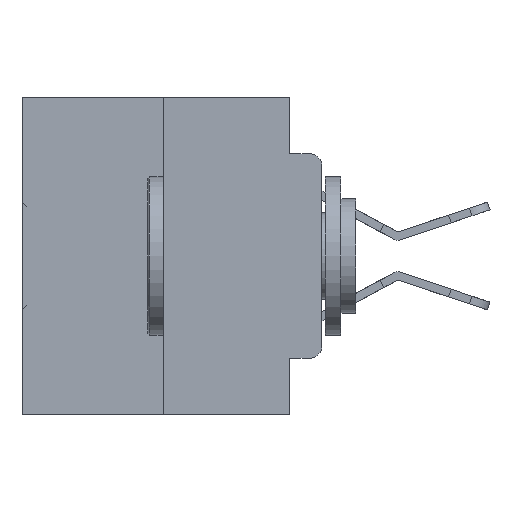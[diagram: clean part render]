
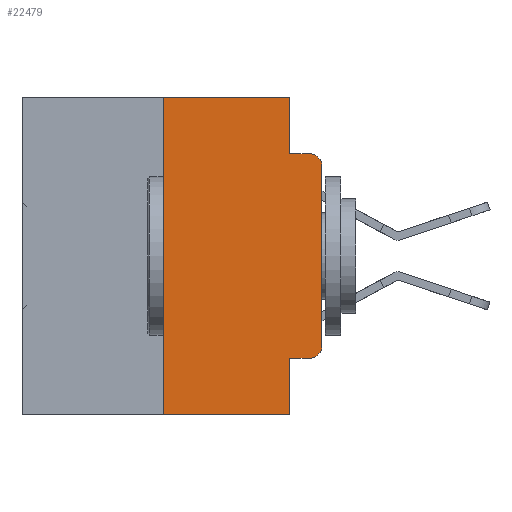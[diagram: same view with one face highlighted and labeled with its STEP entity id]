
A CAD part, left-side view. The second image highlights one B-rep face of the part: STEP entity #22479.
In plain terms, the highlighted planar face has unit normal (-1, 0, 0).
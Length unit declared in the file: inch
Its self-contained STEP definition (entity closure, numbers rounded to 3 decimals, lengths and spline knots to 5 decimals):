
#549 = CARTESIAN_POINT ( 'NONE',  ( 0., 0.473, 0. ) ) ;
#714 = AXIS2_PLACEMENT_3D ( 'NONE', #12423, #21031, #34819 ) ;
#1128 = EDGE_LOOP ( 'NONE', ( #21899, #31407, #31645, #3509, #2574, #10158, #26662, #3017, #32743, #35217 ) ) ;
#1364 = VECTOR ( 'NONE', #4221, 39.37008 ) ;
#1671 = LINE ( 'NONE', #15765, #30282 ) ;
#1735 = VECTOR ( 'NONE', #11716, 39.37008 ) ;
#1980 = VERTEX_POINT ( 'NONE', #30095 ) ;
#2127 = VECTOR ( 'NONE', #31798, 39.37008 ) ;
#2318 = VERTEX_POINT ( 'NONE', #11432 ) ;
#2574 = ORIENTED_EDGE ( 'NONE', *, *, #16960, .F. ) ;
#2674 = AXIS2_PLACEMENT_3D ( 'NONE', #549, #6155, #33897 ) ;
#2813 = VERTEX_POINT ( 'NONE', #35204 ) ;
#3017 = ORIENTED_EDGE ( 'NONE', *, *, #34808, .F. ) ;
#3320 = EDGE_CURVE ( 'NONE', #26210, #14606, #20816, .T. ) ;
#3509 = ORIENTED_EDGE ( 'NONE', *, *, #24870, .F. ) ;
#3551 = DIRECTION ( 'NONE',  ( 0., 0., 1. ) ) ;
#4221 = DIRECTION ( 'NONE',  ( 0., 0., -1. ) ) ;
#4298 = VECTOR ( 'NONE', #3551, 39.37008 ) ;
#4396 = DIRECTION ( 'NONE',  ( -1., 0., 0. ) ) ;
#5252 = CARTESIAN_POINT ( 'NONE',  ( 0., 0.051, 0. ) ) ;
#5351 = VERTEX_POINT ( 'NONE', #15016 ) ;
#5535 = VERTEX_POINT ( 'NONE', #16331 ) ;
#5721 = DIRECTION ( 'NONE',  ( 0., -1., 0. ) ) ;
#6155 = DIRECTION ( 'NONE',  ( 1., 0., 0. ) ) ;
#6475 = LINE ( 'NONE', #14588, #4298 ) ;
#6735 = VERTEX_POINT ( 'NONE', #34587 ) ;
#7124 = DIRECTION ( 'NONE',  ( 0., -1., 0. ) ) ;
#8207 = LINE ( 'NONE', #27161, #15111 ) ;
#8313 = LINE ( 'NONE', #8950, #1364 ) ;
#8692 = CARTESIAN_POINT ( 'NONE',  ( 0., 0.02, -0.0885 ) ) ;
#8950 = CARTESIAN_POINT ( 'NONE',  ( 0., 0.051, 0. ) ) ;
#9137 = LINE ( 'NONE', #31337, #1735 ) ;
#9911 = VECTOR ( 'NONE', #5721, 39.37008 ) ;
#10158 = ORIENTED_EDGE ( 'NONE', *, *, #3320, .F. ) ;
#10572 = DIRECTION ( 'NONE',  ( 0., 0., -1. ) ) ;
#11167 = CARTESIAN_POINT ( 'NONE',  ( 0., 0.051, -0.4115 ) ) ;
#11432 = CARTESIAN_POINT ( 'NONE',  ( 0., 0.051, -0.4115 ) ) ;
#11716 = DIRECTION ( 'NONE',  ( 0., -1., 0. ) ) ;
#12047 = EDGE_CURVE ( 'NONE', #26210, #5351, #9137, .T. ) ;
#12423 = CARTESIAN_POINT ( 'NONE',  ( 0., 0.02, -0.3915 ) ) ;
#12758 = DIRECTION ( 'NONE',  ( 0., 0., -1. ) ) ;
#14368 = VERTEX_POINT ( 'NONE', #8692 ) ;
#14574 = VERTEX_POINT ( 'NONE', #5252 ) ;
#14588 = CARTESIAN_POINT ( 'NONE',  ( 0., 0., 0. ) ) ;
#14606 = VERTEX_POINT ( 'NONE', #20651 ) ;
#14806 = CIRCLE ( 'NONE', #714, 0.02 ) ;
#15016 = CARTESIAN_POINT ( 'NONE',  ( 0., 0.051, -0.5 ) ) ;
#15111 = VECTOR ( 'NONE', #10572, 39.37008 ) ;
#15765 = CARTESIAN_POINT ( 'NONE',  ( 0., 0.051, -0.0885 ) ) ;
#15820 = CARTESIAN_POINT ( 'NONE',  ( 0., 0.25, -0.5 ) ) ;
#16331 = CARTESIAN_POINT ( 'NONE',  ( 0., 0., -0.1085 ) ) ;
#16626 = LINE ( 'NONE', #18146, #31374 ) ;
#16960 = EDGE_CURVE ( 'NONE', #14606, #14574, #16626, .T. ) ;
#17426 = PLANE ( 'NONE',  #2674 ) ;
#18146 = CARTESIAN_POINT ( 'NONE',  ( 0., 0.473, 0. ) ) ;
#20347 = AXIS2_PLACEMENT_3D ( 'NONE', #28985, #4396, #12758 ) ;
#20651 = CARTESIAN_POINT ( 'NONE',  ( 0., 0.25, 0. ) ) ;
#20816 = LINE ( 'NONE', #32272, #2127 ) ;
#20892 = DIRECTION ( 'NONE',  ( 0., -1., 0. ) ) ;
#21031 = DIRECTION ( 'NONE',  ( -1., 0., 0. ) ) ;
#21899 = ORIENTED_EDGE ( 'NONE', *, *, #30699, .T. ) ;
#22479 = ADVANCED_FACE ( 'NONE', ( #30933 ), #17426, .F. ) ;
#24870 = EDGE_CURVE ( 'NONE', #14574, #2813, #8207, .T. ) ;
#25097 = EDGE_CURVE ( 'NONE', #2318, #1980, #31153, .T. ) ;
#26210 = VERTEX_POINT ( 'NONE', #15820 ) ;
#26662 = ORIENTED_EDGE ( 'NONE', *, *, #12047, .T. ) ;
#27161 = CARTESIAN_POINT ( 'NONE',  ( 0., 0.051, 0. ) ) ;
#28985 = CARTESIAN_POINT ( 'NONE',  ( 0., 0.02, -0.1085 ) ) ;
#29090 = EDGE_CURVE ( 'NONE', #5535, #14368, #30031, .T. ) ;
#30031 = CIRCLE ( 'NONE', #20347, 0.02 ) ;
#30095 = CARTESIAN_POINT ( 'NONE',  ( 0., 0.02, -0.4115 ) ) ;
#30282 = VECTOR ( 'NONE', #20892, 39.37008 ) ;
#30699 = EDGE_CURVE ( 'NONE', #6735, #5535, #6475, .T. ) ;
#30933 = FACE_OUTER_BOUND ( 'NONE', #1128, .T. ) ;
#30966 = EDGE_CURVE ( 'NONE', #2813, #14368, #1671, .T. ) ;
#31153 = LINE ( 'NONE', #11167, #9911 ) ;
#31337 = CARTESIAN_POINT ( 'NONE',  ( 0., 0.473, -0.5 ) ) ;
#31374 = VECTOR ( 'NONE', #7124, 39.37008 ) ;
#31407 = ORIENTED_EDGE ( 'NONE', *, *, #29090, .T. ) ;
#31645 = ORIENTED_EDGE ( 'NONE', *, *, #30966, .F. ) ;
#31798 = DIRECTION ( 'NONE',  ( 0., 0., 1. ) ) ;
#32272 = CARTESIAN_POINT ( 'NONE',  ( 0., 0.25, 0. ) ) ;
#32743 = ORIENTED_EDGE ( 'NONE', *, *, #25097, .T. ) ;
#33897 = DIRECTION ( 'NONE',  ( 0., 0., -1. ) ) ;
#34587 = CARTESIAN_POINT ( 'NONE',  ( 0., 0., -0.3915 ) ) ;
#34808 = EDGE_CURVE ( 'NONE', #2318, #5351, #8313, .T. ) ;
#34819 = DIRECTION ( 'NONE',  ( 0., 0., -1. ) ) ;
#35204 = CARTESIAN_POINT ( 'NONE',  ( 0., 0.051, -0.0885 ) ) ;
#35217 = ORIENTED_EDGE ( 'NONE', *, *, #35551, .T. ) ;
#35551 = EDGE_CURVE ( 'NONE', #1980, #6735, #14806, .T. ) ;
